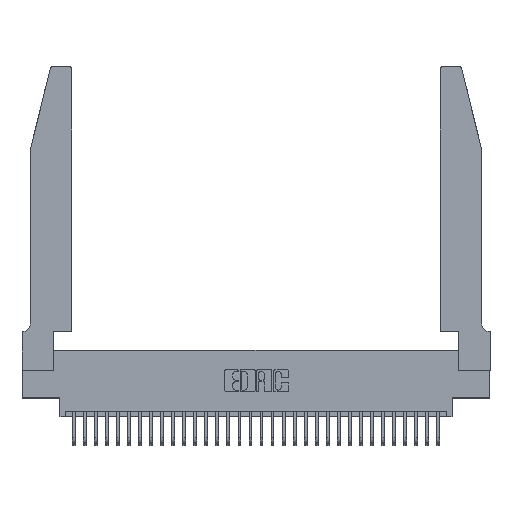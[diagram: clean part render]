
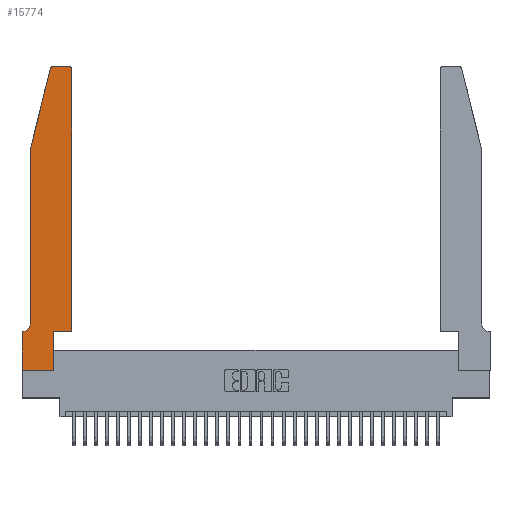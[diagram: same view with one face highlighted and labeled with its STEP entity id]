
A CAD part, top view. The second image highlights one B-rep face of the part: STEP entity #15774.
In plain terms, the highlighted planar face has unit normal (0, 0, 1).
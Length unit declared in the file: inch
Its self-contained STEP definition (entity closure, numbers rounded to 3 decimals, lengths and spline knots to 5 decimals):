
#180 = VERTEX_POINT ( 'NONE', #10770 ) ;
#403 = FACE_OUTER_BOUND ( 'NONE', #26999, .T. ) ;
#1123 = CARTESIAN_POINT ( 'NONE',  ( 0.4505, 0.35, 0.37 ) ) ;
#1508 = LINE ( 'NONE', #18141, #14842 ) ;
#1721 = CIRCLE ( 'NONE', #12246, 0.07 ) ;
#2174 = ORIENTED_EDGE ( 'NONE', *, *, #30033, .T. ) ;
#2562 = VECTOR ( 'NONE', #27670, 39.37008 ) ;
#2564 = DIRECTION ( 'NONE',  ( 1., 0., 0. ) ) ;
#2759 = DIRECTION ( 'NONE',  ( 0., -1., 0. ) ) ;
#3534 = DIRECTION ( 'NONE',  ( 0., 0., -1. ) ) ;
#4062 = CARTESIAN_POINT ( 'NONE',  ( 0.4205, 2.75, 0.37 ) ) ;
#5132 = EDGE_CURVE ( 'NONE', #19637, #19694, #25905, .T. ) ;
#5680 = ORIENTED_EDGE ( 'NONE', *, *, #29909, .T. ) ;
#6214 = CARTESIAN_POINT ( 'NONE',  ( 0.0755, 2., 0.37 ) ) ;
#6852 = LINE ( 'NONE', #6214, #19279 ) ;
#6910 = CARTESIAN_POINT ( 'NONE',  ( 0., 0.35, 0.37 ) ) ;
#7395 = CARTESIAN_POINT ( 'NONE',  ( 0.0755, 0.42, 0.37 ) ) ;
#7530 = VERTEX_POINT ( 'NONE', #7395 ) ;
#8048 = CARTESIAN_POINT ( 'NONE',  ( 0.4205, 2.72, 0.37 ) ) ;
#8214 = AXIS2_PLACEMENT_3D ( 'NONE', #8048, #26567, #10706 ) ;
#9136 = EDGE_CURVE ( 'NONE', #19694, #23794, #22564, .T. ) ;
#9275 = ORIENTED_EDGE ( 'NONE', *, *, #30874, .T. ) ;
#9599 = DIRECTION ( 'NONE',  ( 1., 0., 0. ) ) ;
#9667 = LINE ( 'NONE', #1123, #2562 ) ;
#9804 = VECTOR ( 'NONE', #2759, 39.37008 ) ;
#10479 = VECTOR ( 'NONE', #32994, 39.37008 ) ;
#10706 = DIRECTION ( 'NONE',  ( 1., 0., 0. ) ) ;
#10770 = CARTESIAN_POINT ( 'NONE',  ( 0., 0.35, 0.37 ) ) ;
#11348 = DIRECTION ( 'NONE',  ( 0., 0., 1. ) ) ;
#12246 = AXIS2_PLACEMENT_3D ( 'NONE', #19416, #3534, #22087 ) ;
#12308 = VECTOR ( 'NONE', #2564, 39.37008 ) ;
#13449 = DIRECTION ( 'NONE',  ( 0., 1., 0. ) ) ;
#14222 = AXIS2_PLACEMENT_3D ( 'NONE', #27214, #11348, #29841 ) ;
#14494 = CARTESIAN_POINT ( 'NONE',  ( 0., 0., 0.37 ) ) ;
#14498 = EDGE_CURVE ( 'NONE', #28994, #26065, #9667, .T. ) ;
#14516 = EDGE_CURVE ( 'NONE', #24997, #26033, #16698, .T. ) ;
#14842 = VECTOR ( 'NONE', #26113, 39.37008 ) ;
#15356 = CARTESIAN_POINT ( 'NONE',  ( 0.0755, 2., 0.37 ) ) ;
#15546 = CARTESIAN_POINT ( 'NONE',  ( 0.4505, 2.72, 0.37 ) ) ;
#15774 = ADVANCED_FACE ( 'NONE', ( #403 ), #22785, .T. ) ;
#15825 = CARTESIAN_POINT ( 'NONE',  ( 0.4505, 0.35, 0.37 ) ) ;
#16414 = LINE ( 'NONE', #31962, #21792 ) ;
#16484 = ORIENTED_EDGE ( 'NONE', *, *, #27131, .T. ) ;
#16643 = DIRECTION ( 'NONE',  ( -1., 0., 0. ) ) ;
#16698 = LINE ( 'NONE', #14494, #10479 ) ;
#16792 = VECTOR ( 'NONE', #18017, 39.37008 ) ;
#16831 = LINE ( 'NONE', #18670, #9804 ) ;
#17367 = ORIENTED_EDGE ( 'NONE', *, *, #9136, .T. ) ;
#17377 = CARTESIAN_POINT ( 'NONE',  ( 0.4505, 0.35, 0.37 ) ) ;
#17645 = LINE ( 'NONE', #15356, #16792 ) ;
#17801 = CARTESIAN_POINT ( 'NONE',  ( 0.0055, 0.35, 0.37 ) ) ;
#18017 = DIRECTION ( 'NONE',  ( -0.239, -0.971, 0. ) ) ;
#18141 = CARTESIAN_POINT ( 'NONE',  ( 0.0755, 0.35, 0.37 ) ) ;
#18499 = EDGE_CURVE ( 'NONE', #180, #24997, #16831, .T. ) ;
#18590 = CARTESIAN_POINT ( 'NONE',  ( 0.2865, 0.35, 0.37 ) ) ;
#18670 = CARTESIAN_POINT ( 'NONE',  ( 0., 0., 0.37 ) ) ;
#18885 = EDGE_CURVE ( 'NONE', #33705, #7530, #6852, .T. ) ;
#19279 = VECTOR ( 'NONE', #27409, 39.37008 ) ;
#19318 = VERTEX_POINT ( 'NONE', #18590 ) ;
#19416 = CARTESIAN_POINT ( 'NONE',  ( 0.0055, 0.42, 0.37 ) ) ;
#19637 = VERTEX_POINT ( 'NONE', #4062 ) ;
#19694 = VERTEX_POINT ( 'NONE', #25408 ) ;
#20329 = ORIENTED_EDGE ( 'NONE', *, *, #18499, .T. ) ;
#20750 = ORIENTED_EDGE ( 'NONE', *, *, #14516, .T. ) ;
#21792 = VECTOR ( 'NONE', #13449, 39.37008 ) ;
#21852 = LINE ( 'NONE', #15825, #12308 ) ;
#22087 = DIRECTION ( 'NONE',  ( -1., 0., 0. ) ) ;
#22260 = EDGE_CURVE ( 'NONE', #7530, #29888, #1721, .T. ) ;
#22564 = CIRCLE ( 'NONE', #14222, 0.03 ) ;
#22785 = PLANE ( 'NONE',  #31853 ) ;
#23188 = CARTESIAN_POINT ( 'NONE',  ( 0.25487, 2.72718, 0.37 ) ) ;
#23794 = VERTEX_POINT ( 'NONE', #23188 ) ;
#23886 = ORIENTED_EDGE ( 'NONE', *, *, #18885, .T. ) ;
#24997 = VERTEX_POINT ( 'NONE', #32132 ) ;
#25250 = CARTESIAN_POINT ( 'NONE',  ( 0.0755, 2., 0.37 ) ) ;
#25408 = CARTESIAN_POINT ( 'NONE',  ( 0.284, 2.75, 0.37 ) ) ;
#25449 = DIRECTION ( 'NONE',  ( 0., 0., 1. ) ) ;
#25585 = CIRCLE ( 'NONE', #8214, 0.03 ) ;
#25905 = LINE ( 'NONE', #27170, #32095 ) ;
#26033 = VERTEX_POINT ( 'NONE', #33912 ) ;
#26065 = VERTEX_POINT ( 'NONE', #15546 ) ;
#26113 = DIRECTION ( 'NONE',  ( -1., 0., 0. ) ) ;
#26567 = DIRECTION ( 'NONE',  ( 0., 0., 1. ) ) ;
#26701 = ORIENTED_EDGE ( 'NONE', *, *, #29985, .T. ) ;
#26999 = EDGE_LOOP ( 'NONE', ( #30549, #17367, #16484, #23886, #27723, #5680, #20329, #20750, #9275, #26701, #28298, #2174 ) ) ;
#27131 = EDGE_CURVE ( 'NONE', #23794, #33705, #17645, .T. ) ;
#27170 = CARTESIAN_POINT ( 'NONE',  ( 0.2605, 2.75, 0.37 ) ) ;
#27214 = CARTESIAN_POINT ( 'NONE',  ( 0.284, 2.72, 0.37 ) ) ;
#27409 = DIRECTION ( 'NONE',  ( 0., -1., 0. ) ) ;
#27670 = DIRECTION ( 'NONE',  ( 0., 1., 0. ) ) ;
#27723 = ORIENTED_EDGE ( 'NONE', *, *, #22260, .T. ) ;
#28298 = ORIENTED_EDGE ( 'NONE', *, *, #14498, .T. ) ;
#28994 = VERTEX_POINT ( 'NONE', #17377 ) ;
#29841 = DIRECTION ( 'NONE',  ( 1., 0., 0. ) ) ;
#29888 = VERTEX_POINT ( 'NONE', #17801 ) ;
#29909 = EDGE_CURVE ( 'NONE', #29888, #180, #1508, .T. ) ;
#29985 = EDGE_CURVE ( 'NONE', #19318, #28994, #21852, .T. ) ;
#30033 = EDGE_CURVE ( 'NONE', #26065, #19637, #25585, .T. ) ;
#30549 = ORIENTED_EDGE ( 'NONE', *, *, #5132, .T. ) ;
#30874 = EDGE_CURVE ( 'NONE', #26033, #19318, #16414, .T. ) ;
#31853 = AXIS2_PLACEMENT_3D ( 'NONE', #6910, #25449, #9599 ) ;
#31962 = CARTESIAN_POINT ( 'NONE',  ( 0.2865, 0.35, 0.37 ) ) ;
#32095 = VECTOR ( 'NONE', #16643, 39.37008 ) ;
#32132 = CARTESIAN_POINT ( 'NONE',  ( 0., 0., 0.37 ) ) ;
#32994 = DIRECTION ( 'NONE',  ( 1., 0., 0. ) ) ;
#33705 = VERTEX_POINT ( 'NONE', #25250 ) ;
#33912 = CARTESIAN_POINT ( 'NONE',  ( 0.2865, 0., 0.37 ) ) ;
